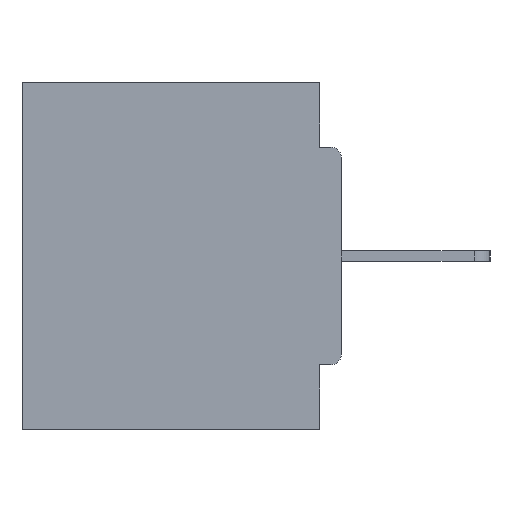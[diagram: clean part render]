
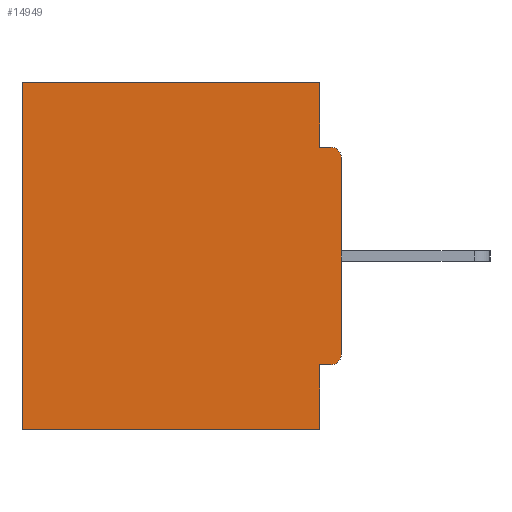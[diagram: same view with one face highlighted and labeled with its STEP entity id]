
A CAD part, left-side view. The second image highlights one B-rep face of the part: STEP entity #14949.
In plain terms, the highlighted planar face has unit normal (-1, 0, 0).
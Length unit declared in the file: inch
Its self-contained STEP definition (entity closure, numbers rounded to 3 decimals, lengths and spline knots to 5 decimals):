
#205 = DIRECTION ( 'NONE',  ( 0., 0., -1. ) ) ;
#556 = EDGE_CURVE ( 'NONE', #24654, #23846, #26322, .T. ) ;
#804 = FACE_OUTER_BOUND ( 'NONE', #27380, .T. ) ;
#1378 = EDGE_CURVE ( 'NONE', #23223, #12012, #4606, .T. ) ;
#1797 = CIRCLE ( 'NONE', #23204, 0.015 ) ;
#1901 = EDGE_CURVE ( 'NONE', #20401, #19219, #12382, .T. ) ;
#2177 = ORIENTED_EDGE ( 'NONE', *, *, #1378, .T. ) ;
#2201 = AXIS2_PLACEMENT_3D ( 'NONE', #5406, #16170, #20490 ) ;
#2433 = DIRECTION ( 'NONE',  ( -1., 0., 0. ) ) ;
#2451 = CARTESIAN_POINT ( 'NONE',  ( 0.298, 0., -0.5 ) ) ;
#2499 = LINE ( 'NONE', #21759, #27537 ) ;
#2732 = CIRCLE ( 'NONE', #3193, 0.015 ) ;
#3193 = AXIS2_PLACEMENT_3D ( 'NONE', #22731, #18396, #12149 ) ;
#3578 = VECTOR ( 'NONE', #25932, 39.37008 ) ;
#3766 = VECTOR ( 'NONE', #12812, 39.37008 ) ;
#3832 = CARTESIAN_POINT ( 'NONE',  ( 0.298, 0., -0.4065 ) ) ;
#4144 = EDGE_CURVE ( 'NONE', #20401, #26999, #2732, .T. ) ;
#4606 = LINE ( 'NONE', #15516, #19339 ) ;
#5406 = CARTESIAN_POINT ( 'NONE',  ( 0.298, 0., 0. ) ) ;
#5960 = EDGE_CURVE ( 'NONE', #12012, #23846, #13630, .T. ) ;
#6192 = CARTESIAN_POINT ( 'NONE',  ( 0.298, 0.46, -0.5 ) ) ;
#6774 = VERTEX_POINT ( 'NONE', #21036 ) ;
#7190 = DIRECTION ( 'NONE',  ( 0., 0., -1. ) ) ;
#7947 = ORIENTED_EDGE ( 'NONE', *, *, #4144, .T. ) ;
#7990 = DIRECTION ( 'NONE',  ( 0., -1., 0. ) ) ;
#8181 = LINE ( 'NONE', #19205, #3766 ) ;
#8543 = LINE ( 'NONE', #17063, #24580 ) ;
#9425 = CARTESIAN_POINT ( 'NONE',  ( 0.298, 0.46, 0. ) ) ;
#9444 = CARTESIAN_POINT ( 'NONE',  ( 0.298, 0.015, -0.0935 ) ) ;
#10216 = EDGE_CURVE ( 'NONE', #19219, #24654, #17797, .T. ) ;
#10597 = ORIENTED_EDGE ( 'NONE', *, *, #1901, .F. ) ;
#11573 = PLANE ( 'NONE',  #2201 ) ;
#11962 = ORIENTED_EDGE ( 'NONE', *, *, #23505, .F. ) ;
#12012 = VERTEX_POINT ( 'NONE', #24049 ) ;
#12149 = DIRECTION ( 'NONE',  ( 0., 0., -1. ) ) ;
#12382 = LINE ( 'NONE', #3832, #25815 ) ;
#12812 = DIRECTION ( 'NONE',  ( 0., 0., -1. ) ) ;
#13630 = LINE ( 'NONE', #9425, #23958 ) ;
#14275 = VERTEX_POINT ( 'NONE', #14600 ) ;
#14600 = CARTESIAN_POINT ( 'NONE',  ( 0.298, 0., -0.1085 ) ) ;
#14603 = ORIENTED_EDGE ( 'NONE', *, *, #16881, .T. ) ;
#14949 = ADVANCED_FACE ( 'NONE', ( #804 ), #11573, .F. ) ;
#15516 = CARTESIAN_POINT ( 'NONE',  ( 0.298, 0., 0. ) ) ;
#15622 = DIRECTION ( 'NONE',  ( 0., 1., 0. ) ) ;
#16170 = DIRECTION ( 'NONE',  ( 1., 0., 0. ) ) ;
#16368 = ORIENTED_EDGE ( 'NONE', *, *, #20153, .F. ) ;
#16401 = ORIENTED_EDGE ( 'NONE', *, *, #10216, .F. ) ;
#16881 = EDGE_CURVE ( 'NONE', #14275, #23266, #1797, .T. ) ;
#17063 = CARTESIAN_POINT ( 'NONE',  ( 0.298, 0., -0.0935 ) ) ;
#17113 = CARTESIAN_POINT ( 'NONE',  ( 0.298, 0.015, -0.1085 ) ) ;
#17200 = DIRECTION ( 'NONE',  ( 0., 1., 0. ) ) ;
#17321 = DIRECTION ( 'NONE',  ( 0., 0., -1. ) ) ;
#17685 = CARTESIAN_POINT ( 'NONE',  ( 0.298, 0.031, 0. ) ) ;
#17797 = LINE ( 'NONE', #26315, #19031 ) ;
#17995 = CARTESIAN_POINT ( 'NONE',  ( 0.298, 0.031, -0.4065 ) ) ;
#18324 = ORIENTED_EDGE ( 'NONE', *, *, #5960, .T. ) ;
#18396 = DIRECTION ( 'NONE',  ( -1., 0., 0. ) ) ;
#19031 = VECTOR ( 'NONE', #7190, 39.37008 ) ;
#19205 = CARTESIAN_POINT ( 'NONE',  ( 0.298, 0., 0. ) ) ;
#19219 = VERTEX_POINT ( 'NONE', #17995 ) ;
#19339 = VECTOR ( 'NONE', #17200, 39.37008 ) ;
#19972 = CARTESIAN_POINT ( 'NONE',  ( 0.298, 0., -0.3915 ) ) ;
#20153 = EDGE_CURVE ( 'NONE', #6774, #23266, #8543, .T. ) ;
#20401 = VERTEX_POINT ( 'NONE', #22325 ) ;
#20490 = DIRECTION ( 'NONE',  ( 0., 0., -1. ) ) ;
#21036 = CARTESIAN_POINT ( 'NONE',  ( 0.298, 0.031, -0.0935 ) ) ;
#21759 = CARTESIAN_POINT ( 'NONE',  ( 0.298, 0.031, -0.5 ) ) ;
#22325 = CARTESIAN_POINT ( 'NONE',  ( 0.298, 0.015, -0.4065 ) ) ;
#22731 = CARTESIAN_POINT ( 'NONE',  ( 0.298, 0.015, -0.3915 ) ) ;
#23008 = CARTESIAN_POINT ( 'NONE',  ( 0.298, 0.031, -0.5 ) ) ;
#23016 = ORIENTED_EDGE ( 'NONE', *, *, #27266, .F. ) ;
#23204 = AXIS2_PLACEMENT_3D ( 'NONE', #17113, #2433, #205 ) ;
#23223 = VERTEX_POINT ( 'NONE', #17685 ) ;
#23266 = VERTEX_POINT ( 'NONE', #9444 ) ;
#23505 = EDGE_CURVE ( 'NONE', #14275, #26999, #8181, .T. ) ;
#23846 = VERTEX_POINT ( 'NONE', #6192 ) ;
#23958 = VECTOR ( 'NONE', #26452, 39.37008 ) ;
#24049 = CARTESIAN_POINT ( 'NONE',  ( 0.298, 0.46, 0. ) ) ;
#24580 = VECTOR ( 'NONE', #7990, 39.37008 ) ;
#24654 = VERTEX_POINT ( 'NONE', #23008 ) ;
#25815 = VECTOR ( 'NONE', #15622, 39.37008 ) ;
#25932 = DIRECTION ( 'NONE',  ( 0., 1., 0. ) ) ;
#26315 = CARTESIAN_POINT ( 'NONE',  ( 0.298, 0.031, -0.5 ) ) ;
#26322 = LINE ( 'NONE', #2451, #3578 ) ;
#26452 = DIRECTION ( 'NONE',  ( 0., 0., -1. ) ) ;
#26703 = ORIENTED_EDGE ( 'NONE', *, *, #556, .F. ) ;
#26999 = VERTEX_POINT ( 'NONE', #19972 ) ;
#27266 = EDGE_CURVE ( 'NONE', #23223, #6774, #2499, .T. ) ;
#27380 = EDGE_LOOP ( 'NONE', ( #14603, #16368, #23016, #2177, #18324, #26703, #16401, #10597, #7947, #11962 ) ) ;
#27537 = VECTOR ( 'NONE', #17321, 39.37008 ) ;
